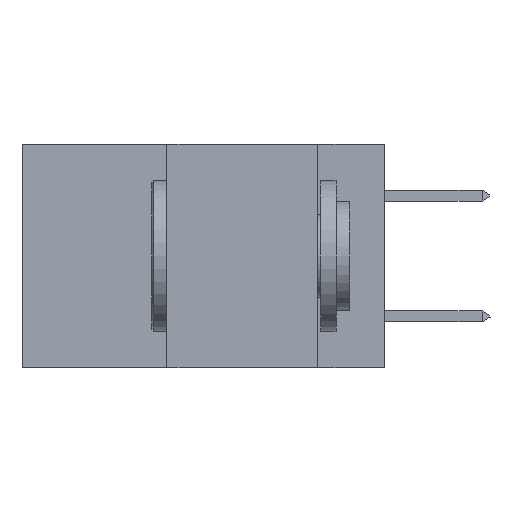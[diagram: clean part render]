
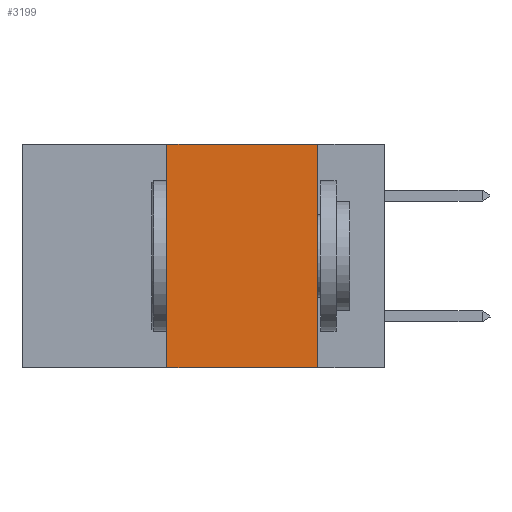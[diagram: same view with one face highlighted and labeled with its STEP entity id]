
A CAD part, left-side view. The second image highlights one B-rep face of the part: STEP entity #3199.
In plain terms, the highlighted planar face has unit normal (-1, 0, 0).
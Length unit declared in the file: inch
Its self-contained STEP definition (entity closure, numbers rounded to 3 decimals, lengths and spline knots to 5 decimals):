
#159 = VECTOR ( 'NONE', #10446, 39.37008 ) ;
#266 = EDGE_LOOP ( 'NONE', ( #2304, #1097, #406, #7145 ) ) ;
#349 = VECTOR ( 'NONE', #10403, 39.37008 ) ;
#406 = ORIENTED_EDGE ( 'NONE', *, *, #6766, .F. ) ;
#643 = LINE ( 'NONE', #4982, #349 ) ;
#1097 = ORIENTED_EDGE ( 'NONE', *, *, #10553, .F. ) ;
#1251 = VECTOR ( 'NONE', #5917, 39.37008 ) ;
#1509 = CARTESIAN_POINT ( 'NONE',  ( 0., 0.36, -0.37 ) ) ;
#1634 = DIRECTION ( 'NONE',  ( 0., 0., -1. ) ) ;
#2158 = VECTOR ( 'NONE', #3495, 39.37008 ) ;
#2304 = ORIENTED_EDGE ( 'NONE', *, *, #8675, .F. ) ;
#2457 = LINE ( 'NONE', #6249, #2158 ) ;
#2571 = AXIS2_PLACEMENT_3D ( 'NONE', #11601, #7068, #1634 ) ;
#2576 = LINE ( 'NONE', #7721, #159 ) ;
#3035 = EDGE_CURVE ( 'NONE', #9500, #5530, #2576, .T. ) ;
#3199 = ADVANCED_FACE ( 'NONE', ( #10400 ), #6172, .F. ) ;
#3424 = CARTESIAN_POINT ( 'NONE',  ( 0., 0.11, -0.37 ) ) ;
#3495 = DIRECTION ( 'NONE',  ( 0., 0., 1. ) ) ;
#4964 = CARTESIAN_POINT ( 'NONE',  ( 0., 0.11, 0. ) ) ;
#4982 = CARTESIAN_POINT ( 'NONE',  ( 0., 0.6, 0. ) ) ;
#5530 = VERTEX_POINT ( 'NONE', #3424 ) ;
#5917 = DIRECTION ( 'NONE',  ( 0., 0., -1. ) ) ;
#6097 = LINE ( 'NONE', #7690, #1251 ) ;
#6172 = PLANE ( 'NONE',  #2571 ) ;
#6249 = CARTESIAN_POINT ( 'NONE',  ( 0., 0.36, 0. ) ) ;
#6766 = EDGE_CURVE ( 'NONE', #9500, #11564, #2457, .T. ) ;
#7068 = DIRECTION ( 'NONE',  ( 1., 0., 0. ) ) ;
#7145 = ORIENTED_EDGE ( 'NONE', *, *, #3035, .T. ) ;
#7690 = CARTESIAN_POINT ( 'NONE',  ( 0., 0.11, 0. ) ) ;
#7721 = CARTESIAN_POINT ( 'NONE',  ( 0., 0.6, -0.37 ) ) ;
#8675 = EDGE_CURVE ( 'NONE', #9387, #5530, #6097, .T. ) ;
#9387 = VERTEX_POINT ( 'NONE', #4964 ) ;
#9500 = VERTEX_POINT ( 'NONE', #1509 ) ;
#10400 = FACE_OUTER_BOUND ( 'NONE', #266, .T. ) ;
#10403 = DIRECTION ( 'NONE',  ( 0., -1., 0. ) ) ;
#10446 = DIRECTION ( 'NONE',  ( 0., -1., 0. ) ) ;
#10553 = EDGE_CURVE ( 'NONE', #11564, #9387, #643, .T. ) ;
#11480 = CARTESIAN_POINT ( 'NONE',  ( 0., 0.36, 0. ) ) ;
#11564 = VERTEX_POINT ( 'NONE', #11480 ) ;
#11601 = CARTESIAN_POINT ( 'NONE',  ( 0., 0.6, 0. ) ) ;
